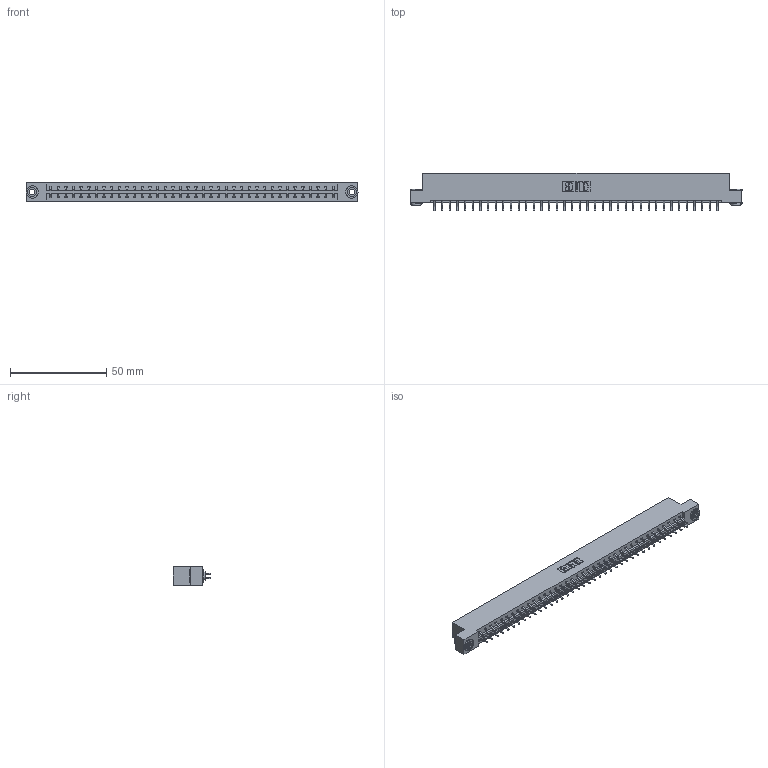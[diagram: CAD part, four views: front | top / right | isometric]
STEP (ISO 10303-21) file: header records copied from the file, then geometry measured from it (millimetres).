
FILE_DESCRIPTION (( 'STEP AP203' ), '1' );
FILE_NAME ('833-076-556-203.STEP', '2020-06-05T18:53:15', ( '' ), ( '' ), 'SwSTEP 2.0', 'SolidWorks 2020', '' );
FILE_SCHEMA (( 'CONFIG_CONTROL_DESIGN' ));
Length unit declared in the file: inch
Products named in the file (4): 833-076-556-203; 833 Part_Flush - .156 Dia - TH; 345-250-002_345-250-002-102; 345-292-001_556 Tail
Assembly tree (79 placements, depth 2):
  833-076-556-203
    833 Part_Flush - .156 Dia - TH
    345-292-001_556 Tail  x76
    345-250-002_345-250-002-102  x2
Bounding box: 172.11 x 19.57 x 9.4 mm (x, y, z)
Volume: 17550.5 mm3; surface area: 20852 mm2
Topology: 79 solids, 79 shells, 4560 faces, 13535 edges, 8918 vertices
Faces by surface type: plane 3120, cylinder 1432, cone 8
Entity records: 25834 total; most frequent: CARTESIAN_POINT 4277, ORIENTED_EDGE 4194, DIRECTION 3683, EDGE_CURVE 2097, LINE 1937, VECTOR 1937, VERTEX_POINT 1394, AXIS2_PLACEMENT_3D 873
